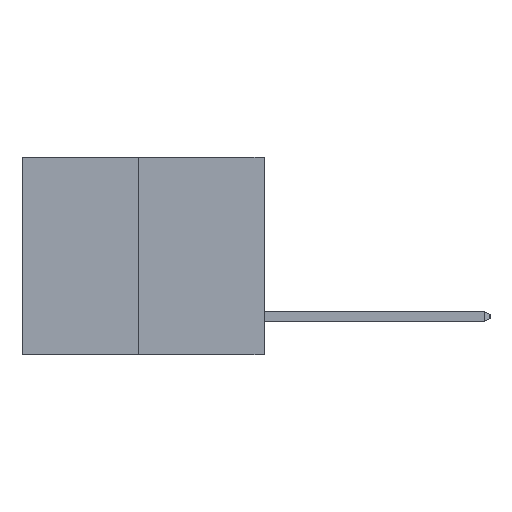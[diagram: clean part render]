
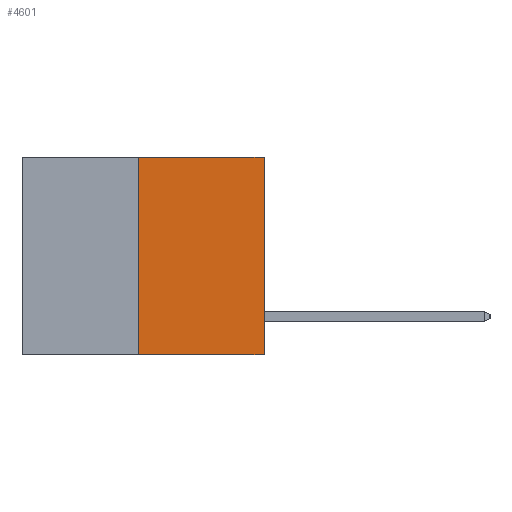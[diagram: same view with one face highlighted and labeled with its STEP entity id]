
A CAD part, left-side view. The second image highlights one B-rep face of the part: STEP entity #4601.
In plain terms, the highlighted planar face has unit normal (-1, 0, 0).
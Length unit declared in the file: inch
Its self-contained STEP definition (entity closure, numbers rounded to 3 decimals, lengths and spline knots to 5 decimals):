
#327 = LINE ( 'NONE', #6125, #5665 ) ;
#667 = DIRECTION ( 'NONE',  ( 0., 0., 1. ) ) ;
#1035 = VECTOR ( 'NONE', #4801, 39.37008 ) ;
#1408 = VECTOR ( 'NONE', #667, 39.37008 ) ;
#1920 = ORIENTED_EDGE ( 'NONE', *, *, #3240, .F. ) ;
#2939 = VERTEX_POINT ( 'NONE', #9771 ) ;
#3240 = EDGE_CURVE ( 'NONE', #5663, #2939, #327, .T. ) ;
#4279 = CARTESIAN_POINT ( 'NONE',  ( 0., 0.312, -0.49 ) ) ;
#4323 = CARTESIAN_POINT ( 'NONE',  ( 0., 0.312, 0. ) ) ;
#4601 = ADVANCED_FACE ( 'NONE', ( #13204 ), #9398, .F. ) ;
#4801 = DIRECTION ( 'NONE',  ( 0., 0., 1. ) ) ;
#5136 = DIRECTION ( 'NONE',  ( 1., 0., 0. ) ) ;
#5289 = LINE ( 'NONE', #13033, #8837 ) ;
#5663 = VERTEX_POINT ( 'NONE', #4323 ) ;
#5665 = VECTOR ( 'NONE', #8206, 39.37008 ) ;
#5779 = AXIS2_PLACEMENT_3D ( 'NONE', #6176, #5136, #12732 ) ;
#6125 = CARTESIAN_POINT ( 'NONE',  ( 0., 0.6, 0. ) ) ;
#6176 = CARTESIAN_POINT ( 'NONE',  ( 0., 0.6, 0. ) ) ;
#6704 = LINE ( 'NONE', #11022, #1035 ) ;
#6996 = CARTESIAN_POINT ( 'NONE',  ( 0., 0.312, -0.49 ) ) ;
#7595 = EDGE_LOOP ( 'NONE', ( #9633, #8895, #13429, #1920 ) ) ;
#7776 = VERTEX_POINT ( 'NONE', #12750 ) ;
#8206 = DIRECTION ( 'NONE',  ( 0., -1., 0. ) ) ;
#8837 = VECTOR ( 'NONE', #9873, 39.37008 ) ;
#8895 = ORIENTED_EDGE ( 'NONE', *, *, #12557, .T. ) ;
#9398 = PLANE ( 'NONE',  #5779 ) ;
#9633 = ORIENTED_EDGE ( 'NONE', *, *, #10124, .F. ) ;
#9771 = CARTESIAN_POINT ( 'NONE',  ( 0., 0., 0. ) ) ;
#9873 = DIRECTION ( 'NONE',  ( 0., -1., 0. ) ) ;
#10124 = EDGE_CURVE ( 'NONE', #11067, #5663, #12152, .T. ) ;
#11022 = CARTESIAN_POINT ( 'NONE',  ( 0., 0., 0. ) ) ;
#11067 = VERTEX_POINT ( 'NONE', #4279 ) ;
#11561 = EDGE_CURVE ( 'NONE', #7776, #2939, #6704, .T. ) ;
#12152 = LINE ( 'NONE', #6996, #1408 ) ;
#12557 = EDGE_CURVE ( 'NONE', #11067, #7776, #5289, .T. ) ;
#12732 = DIRECTION ( 'NONE',  ( 0., 0., -1. ) ) ;
#12750 = CARTESIAN_POINT ( 'NONE',  ( 0., 0., -0.49 ) ) ;
#13033 = CARTESIAN_POINT ( 'NONE',  ( 0., 0.6, -0.49 ) ) ;
#13204 = FACE_OUTER_BOUND ( 'NONE', #7595, .T. ) ;
#13429 = ORIENTED_EDGE ( 'NONE', *, *, #11561, .T. ) ;
